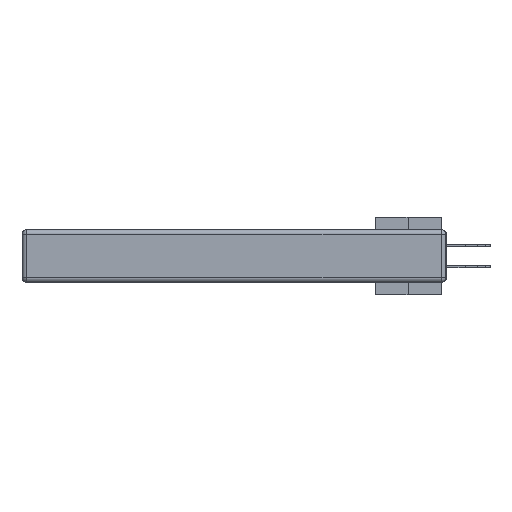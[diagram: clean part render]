
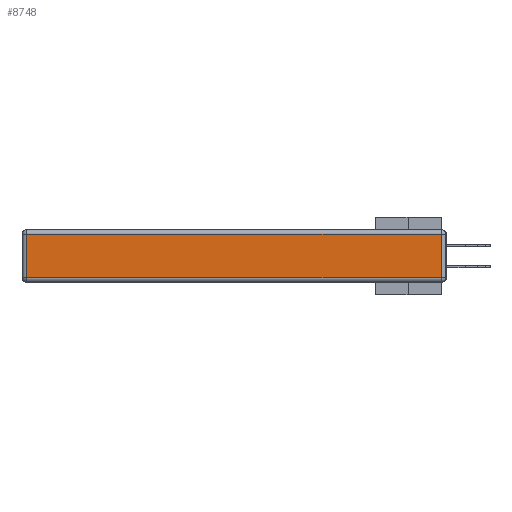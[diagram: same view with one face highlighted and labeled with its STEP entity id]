
A CAD part, left-side view. The second image highlights one B-rep face of the part: STEP entity #8748.
In plain terms, the highlighted planar face has unit normal (-1, 0, 0).
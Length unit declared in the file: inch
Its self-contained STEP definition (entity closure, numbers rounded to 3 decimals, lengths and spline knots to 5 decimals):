
#974 = CARTESIAN_POINT ( 'NONE',  ( 0., 0.03, -0.03 ) ) ;
#1293 = VERTEX_POINT ( 'NONE', #29404 ) ;
#1854 = LINE ( 'NONE', #24587, #29131 ) ;
#2603 = EDGE_LOOP ( 'NONE', ( #23943, #15602, #6163, #2657 ) ) ;
#2657 = ORIENTED_EDGE ( 'NONE', *, *, #26711, .T. ) ;
#5472 = CARTESIAN_POINT ( 'NONE',  ( 0., 2.72, -0.03 ) ) ;
#6163 = ORIENTED_EDGE ( 'NONE', *, *, #8448, .T. ) ;
#6508 = VECTOR ( 'NONE', #8733, 39.37008 ) ;
#7016 = CARTESIAN_POINT ( 'NONE',  ( 0., 0., -0.313 ) ) ;
#7193 = DIRECTION ( 'NONE',  ( 0., 0., 1. ) ) ;
#7461 = DIRECTION ( 'NONE',  ( 0., 1., 0. ) ) ;
#7798 = AXIS2_PLACEMENT_3D ( 'NONE', #15062, #26897, #29869 ) ;
#8448 = EDGE_CURVE ( 'NONE', #32412, #27306, #22863, .T. ) ;
#8733 = DIRECTION ( 'NONE',  ( 0., 0., -1. ) ) ;
#8748 = ADVANCED_FACE ( 'NONE', ( #11880 ), #12127, .T. ) ;
#10250 = LINE ( 'NONE', #7016, #17540 ) ;
#11880 = FACE_OUTER_BOUND ( 'NONE', #2603, .T. ) ;
#12127 = PLANE ( 'NONE',  #7798 ) ;
#12572 = EDGE_CURVE ( 'NONE', #29050, #1293, #10250, .T. ) ;
#15062 = CARTESIAN_POINT ( 'NONE',  ( 0., 0., -0.343 ) ) ;
#15602 = ORIENTED_EDGE ( 'NONE', *, *, #28162, .T. ) ;
#17540 = VECTOR ( 'NONE', #33336, 39.37008 ) ;
#17823 = LINE ( 'NONE', #26197, #6508 ) ;
#21953 = VECTOR ( 'NONE', #7461, 39.37008 ) ;
#22863 = LINE ( 'NONE', #24866, #21953 ) ;
#23943 = ORIENTED_EDGE ( 'NONE', *, *, #12572, .T. ) ;
#24587 = CARTESIAN_POINT ( 'NONE',  ( 0., 0.03, -0.343 ) ) ;
#24866 = CARTESIAN_POINT ( 'NONE',  ( 0., 2.75, -0.03 ) ) ;
#26197 = CARTESIAN_POINT ( 'NONE',  ( 0., 2.72, -0.343 ) ) ;
#26711 = EDGE_CURVE ( 'NONE', #27306, #29050, #17823, .T. ) ;
#26897 = DIRECTION ( 'NONE',  ( -1., 0., 0. ) ) ;
#27306 = VERTEX_POINT ( 'NONE', #5472 ) ;
#28162 = EDGE_CURVE ( 'NONE', #1293, #32412, #1854, .T. ) ;
#29050 = VERTEX_POINT ( 'NONE', #34838 ) ;
#29131 = VECTOR ( 'NONE', #7193, 39.37008 ) ;
#29404 = CARTESIAN_POINT ( 'NONE',  ( 0., 0.03, -0.313 ) ) ;
#29869 = DIRECTION ( 'NONE',  ( 0., 0., 1. ) ) ;
#32412 = VERTEX_POINT ( 'NONE', #974 ) ;
#33336 = DIRECTION ( 'NONE',  ( 0., -1., 0. ) ) ;
#34838 = CARTESIAN_POINT ( 'NONE',  ( 0., 2.72, -0.313 ) ) ;
